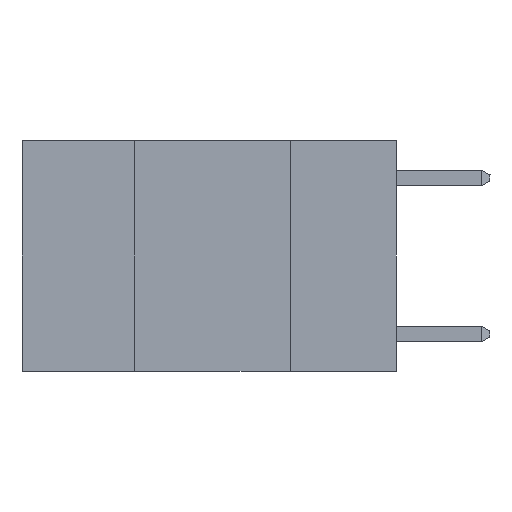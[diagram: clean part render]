
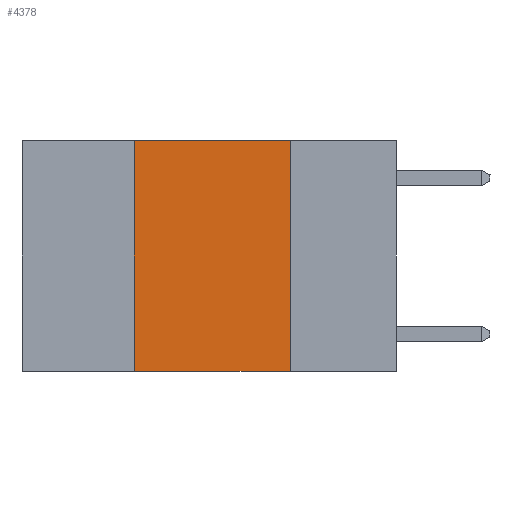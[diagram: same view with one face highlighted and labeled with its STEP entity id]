
A CAD part, left-side view. The second image highlights one B-rep face of the part: STEP entity #4378.
In plain terms, the highlighted planar face has unit normal (-1, 0, 0).
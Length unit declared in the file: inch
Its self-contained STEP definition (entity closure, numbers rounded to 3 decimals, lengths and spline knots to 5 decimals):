
#106 = EDGE_CURVE ( 'NONE', #10375, #5585, #922, .T. ) ;
#324 = EDGE_CURVE ( 'NONE', #7459, #10375, #8614, .T. ) ;
#794 = DIRECTION ( 'NONE',  ( 0., -1., 0. ) ) ;
#922 = LINE ( 'NONE', #1691, #7951 ) ;
#1223 = LINE ( 'NONE', #3644, #10487 ) ;
#1288 = DIRECTION ( 'NONE',  ( 0., 0., -1. ) ) ;
#1675 = DIRECTION ( 'NONE',  ( 0., -1., 0. ) ) ;
#1691 = CARTESIAN_POINT ( 'NONE',  ( 0., 0.6, 0. ) ) ;
#1852 = CARTESIAN_POINT ( 'NONE',  ( 0., 0.42, 0. ) ) ;
#2365 = LINE ( 'NONE', #6959, #11466 ) ;
#2577 = VERTEX_POINT ( 'NONE', #10979 ) ;
#2755 = EDGE_LOOP ( 'NONE', ( #4322, #5248, #5667, #6935 ) ) ;
#3078 = FACE_OUTER_BOUND ( 'NONE', #2755, .T. ) ;
#3590 = CARTESIAN_POINT ( 'NONE',  ( 0., 0.17, 0. ) ) ;
#3644 = CARTESIAN_POINT ( 'NONE',  ( 0., 0.6, -0.37 ) ) ;
#4322 = ORIENTED_EDGE ( 'NONE', *, *, #5372, .F. ) ;
#4346 = CARTESIAN_POINT ( 'NONE',  ( 0., 0.42, 0. ) ) ;
#4378 = ADVANCED_FACE ( 'NONE', ( #3078 ), #9352, .F. ) ;
#4387 = CARTESIAN_POINT ( 'NONE',  ( 0., 0.42, -0.37 ) ) ;
#5248 = ORIENTED_EDGE ( 'NONE', *, *, #106, .F. ) ;
#5372 = EDGE_CURVE ( 'NONE', #5585, #2577, #2365, .T. ) ;
#5585 = VERTEX_POINT ( 'NONE', #3590 ) ;
#5667 = ORIENTED_EDGE ( 'NONE', *, *, #324, .F. ) ;
#5940 = CARTESIAN_POINT ( 'NONE',  ( 0., 0.6, 0. ) ) ;
#6060 = DIRECTION ( 'NONE',  ( 0., 0., -1. ) ) ;
#6826 = DIRECTION ( 'NONE',  ( 1., 0., 0. ) ) ;
#6935 = ORIENTED_EDGE ( 'NONE', *, *, #7964, .T. ) ;
#6959 = CARTESIAN_POINT ( 'NONE',  ( 0., 0.17, 0. ) ) ;
#7459 = VERTEX_POINT ( 'NONE', #4387 ) ;
#7951 = VECTOR ( 'NONE', #1675, 39.37008 ) ;
#7964 = EDGE_CURVE ( 'NONE', #7459, #2577, #1223, .T. ) ;
#8082 = VECTOR ( 'NONE', #10209, 39.37008 ) ;
#8614 = LINE ( 'NONE', #1852, #8082 ) ;
#9352 = PLANE ( 'NONE',  #10308 ) ;
#10209 = DIRECTION ( 'NONE',  ( 0., 0., 1. ) ) ;
#10308 = AXIS2_PLACEMENT_3D ( 'NONE', #5940, #6826, #1288 ) ;
#10375 = VERTEX_POINT ( 'NONE', #4346 ) ;
#10487 = VECTOR ( 'NONE', #794, 39.37008 ) ;
#10979 = CARTESIAN_POINT ( 'NONE',  ( 0., 0.17, -0.37 ) ) ;
#11466 = VECTOR ( 'NONE', #6060, 39.37008 ) ;
